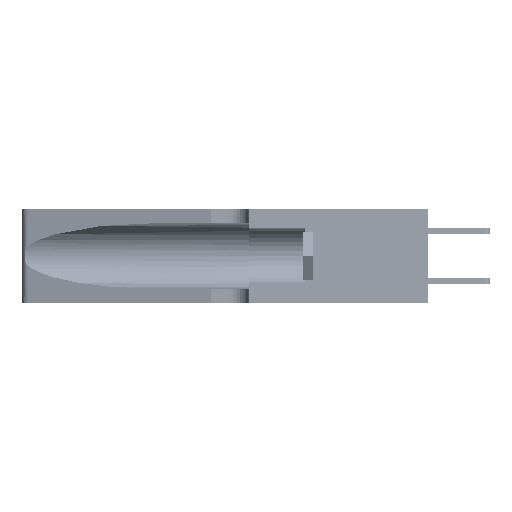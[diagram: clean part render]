
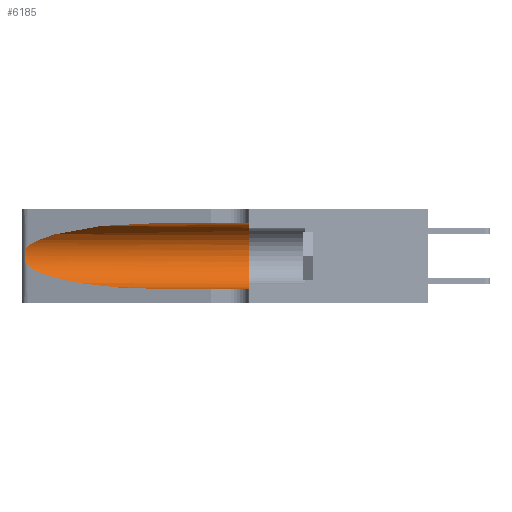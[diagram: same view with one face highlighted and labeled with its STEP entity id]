
A CAD part, left-side view. The second image highlights one B-rep face of the part: STEP entity #6185.
In plain terms, the highlighted cylindrical face has radius 3.308 mm (diameter 6.617 mm), a partial arc.
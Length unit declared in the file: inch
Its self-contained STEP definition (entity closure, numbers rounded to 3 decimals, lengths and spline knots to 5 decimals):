
#1292 = CARTESIAN_POINT ( 'NONE',  ( 0.1305, 0.72297, 0.31525 ) ) ;
#2131 = CIRCLE ( 'NONE', #4792, 0.13025 ) ;
#2577 = CARTESIAN_POINT ( 'NONE',  ( 0.1305, 1.61858, 0.05475 ) ) ;
#3238 = DIRECTION ( 'NONE',  ( 0., -1., 0. ) ) ;
#3683 = ORIENTED_EDGE ( 'NONE', *, *, #45766, .F. ) ;
#4792 = AXIS2_PLACEMENT_3D ( 'NONE', #29390, #17560, #25911 ) ;
#6185 = ADVANCED_FACE ( 'NONE', ( #15358 ), #26576, .F. ) ;
#6269 = CARTESIAN_POINT ( 'NONE',  ( 0.1305, 0.72297, 0.31525 ) ) ;
#6712 = CARTESIAN_POINT ( 'NONE',  ( 0.25854, 1.2359, 0.20912 ) ) ;
#6936 = DIRECTION ( 'NONE',  ( 0., 0., -1. ) ) ;
#7240 = CARTESIAN_POINT ( 'NONE',  ( 0.25789, 1.23486, 0.15765 ) ) ;
#7519 = AXIS2_PLACEMENT_3D ( 'NONE', #14928, #30418, #6936 ) ;
#7957 = EDGE_CURVE ( 'NONE', #50134, #43914, #17342, .T. ) ;
#9458 = CARTESIAN_POINT ( 'NONE',  ( 0.18966, 0.96281, 0.31525 ) ) ;
#10882 = CARTESIAN_POINT ( 'NONE',  ( 0.25487, 1.22718, 0.22369 ) ) ;
#11214 = EDGE_CURVE ( 'NONE', #27951, #50134, #32535, .T. ) ;
#11666 = VERTEX_POINT ( 'NONE', #6269 ) ;
#12472 = DIRECTION ( 'NONE',  ( 0., -1., 0. ) ) ;
#12780 = ORIENTED_EDGE ( 'NONE', *, *, #7957, .T. ) ;
#13883 = EDGE_LOOP ( 'NONE', ( #15069, #44303, #22806, #12780, #3683, #49637 ) ) ;
#14928 = CARTESIAN_POINT ( 'NONE',  ( 0.1305, 1.61858, 0.185 ) ) ;
#15050 = CARTESIAN_POINT ( 'NONE',  ( 0.25787, 1.23484, 0.2124 ) ) ;
#15069 = ORIENTED_EDGE ( 'NONE', *, *, #44984, .T. ) ;
#15358 = FACE_OUTER_BOUND ( 'NONE', #13883, .T. ) ;
#16461 = CARTESIAN_POINT ( 'NONE',  ( 0.1305, 1.61858, 0.31525 ) ) ;
#16710 = LINE ( 'NONE', #16461, #41634 ) ;
#17342 = LINE ( 'NONE', #2577, #44733 ) ;
#17560 = DIRECTION ( 'NONE',  ( 0., 1., 0. ) ) ;
#19072 = CARTESIAN_POINT ( 'NONE',  ( 0.26017, 1.23833, 0.17102 ) ) ;
#19541 = CARTESIAN_POINT ( 'NONE',  ( 0.25487, 1.22718, 0.14631 ) ) ;
#19890 = VERTEX_POINT ( 'NONE', #28133 ) ;
#21103 = CARTESIAN_POINT ( 'NONE',  ( 0.1305, 0.72297, 0.05475 ) ) ;
#21336 = CARTESIAN_POINT ( 'NONE',  ( 0.1305, 0.35, 0.31525 ) ) ;
#22376 = CARTESIAN_POINT ( 'NONE',  ( 0.25639, 1.23184, 0.21858 ) ) ;
#22806 = ORIENTED_EDGE ( 'NONE', *, *, #11214, .T. ) ;
#23069 = CARTESIAN_POINT ( 'NONE',  ( 0.25487, 1.22718, 0.14631 ) ) ;
#23950 = CARTESIAN_POINT ( 'NONE',  ( 0.25487, 1.22718, 0.14631 ) ) ;
#24136 = CARTESIAN_POINT ( 'NONE',  ( 0.1305, 0.35, 0.05475 ) ) ;
#25292 = CARTESIAN_POINT ( 'NONE',  ( 0.2373, 1.15595, 0.28018 ) ) ;
#25911 = DIRECTION ( 'NONE',  ( 0., 0., 1. ) ) ;
#26576 = CYLINDRICAL_SURFACE ( 'NONE', #7519, 0.13025 ) ;
#27070 = CARTESIAN_POINT ( 'NONE',  ( 0.26075, 1.23896, 0.19203 ) ) ;
#27951 = VERTEX_POINT ( 'NONE', #23950 ) ;
#28133 = CARTESIAN_POINT ( 'NONE',  ( 0.25487, 1.22718, 0.22369 ) ) ;
#28290 = VERTEX_POINT ( 'NONE', #21336 ) ;
#29390 = CARTESIAN_POINT ( 'NONE',  ( 0.1305, 0.35, 0.185 ) ) ;
#29622 = CARTESIAN_POINT ( 'NONE',  ( 0.25487, 1.22718, 0.22369 ) ) ;
#30418 = DIRECTION ( 'NONE',  ( 0., -1., 0. ) ) ;
#31683 = CARTESIAN_POINT ( 'NONE',  ( 0.18966, 0.96281, 0.05475 ) ) ;
#31880 = B_SPLINE_CURVE_WITH_KNOTS ( 'NONE', 3,
 ( #10882, #38891, #22376, #15050, #6712, #42895, #27070, #34530, #19072, #46200, #7240, #35058, #42383, #23069 ),
 .UNSPECIFIED., .F., .F.,
 ( 4, 2, 2, 2, 2, 2, 4 ),
 ( 0., 0.00027, 0.00053, 0.00107, 0.0016, 0.00187, 0.00214 ),
 .UNSPECIFIED. ) ;
#32535 =( BOUNDED_CURVE ( )  B_SPLINE_CURVE ( 3, ( #19541, #35366, #31683, #47341 ),
 .UNSPECIFIED., .F., .T. ) 
 B_SPLINE_CURVE_WITH_KNOTS ( ( 4, 4 ),
 ( 3.44316, 4.71239 ),
 .UNSPECIFIED. ) 
 CURVE ( )  GEOMETRIC_REPRESENTATION_ITEM ( )  RATIONAL_B_SPLINE_CURVE ( ( 1., 0.87, 0.87, 1. ) ) 
 REPRESENTATION_ITEM ( '' )  );
#34530 = CARTESIAN_POINT ( 'NONE',  ( 0.26075, 1.23896, 0.178 ) ) ;
#35058 = CARTESIAN_POINT ( 'NONE',  ( 0.25639, 1.23186, 0.15144 ) ) ;
#35366 = CARTESIAN_POINT ( 'NONE',  ( 0.2373, 1.15595, 0.08982 ) ) ;
#38891 = CARTESIAN_POINT ( 'NONE',  ( 0.25555, 1.22994, 0.2215 ) ) ;
#41634 = VECTOR ( 'NONE', #12472, 39.37008 ) ;
#42383 = CARTESIAN_POINT ( 'NONE',  ( 0.25555, 1.22993, 0.14849 ) ) ;
#42539 = EDGE_CURVE ( 'NONE', #19890, #27951, #31880, .T. ) ;
#42895 = CARTESIAN_POINT ( 'NONE',  ( 0.26018, 1.23835, 0.19895 ) ) ;
#43914 = VERTEX_POINT ( 'NONE', #24136 ) ;
#44303 = ORIENTED_EDGE ( 'NONE', *, *, #42539, .T. ) ;
#44733 = VECTOR ( 'NONE', #3238, 39.37008 ) ;
#44984 = EDGE_CURVE ( 'NONE', #11666, #19890, #50993, .T. ) ;
#45766 = EDGE_CURVE ( 'NONE', #28290, #43914, #2131, .T. ) ;
#46200 = CARTESIAN_POINT ( 'NONE',  ( 0.25856, 1.23593, 0.16098 ) ) ;
#47341 = CARTESIAN_POINT ( 'NONE',  ( 0.1305, 0.72297, 0.05475 ) ) ;
#49414 = EDGE_CURVE ( 'NONE', #11666, #28290, #16710, .T. ) ;
#49637 = ORIENTED_EDGE ( 'NONE', *, *, #49414, .F. ) ;
#50134 = VERTEX_POINT ( 'NONE', #21103 ) ;
#50993 =( BOUNDED_CURVE ( )  B_SPLINE_CURVE ( 3, ( #1292, #9458, #25292, #29622 ),
 .UNSPECIFIED., .F., .T. ) 
 B_SPLINE_CURVE_WITH_KNOTS ( ( 4, 4 ),
 ( 1.5708, 2.84003 ),
 .UNSPECIFIED. ) 
 CURVE ( )  GEOMETRIC_REPRESENTATION_ITEM ( )  RATIONAL_B_SPLINE_CURVE ( ( 1., 0.87, 0.87, 1. ) ) 
 REPRESENTATION_ITEM ( '' )  );
